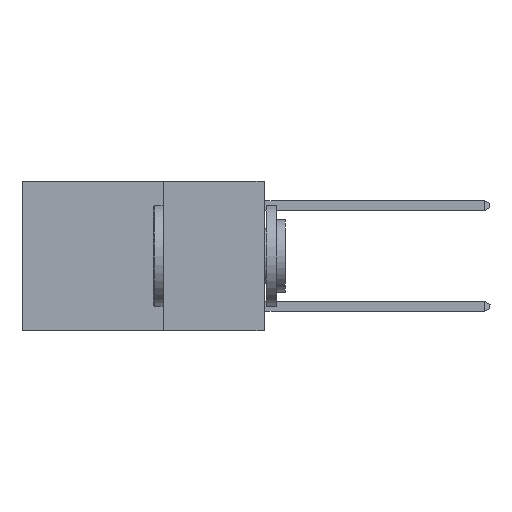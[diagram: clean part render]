
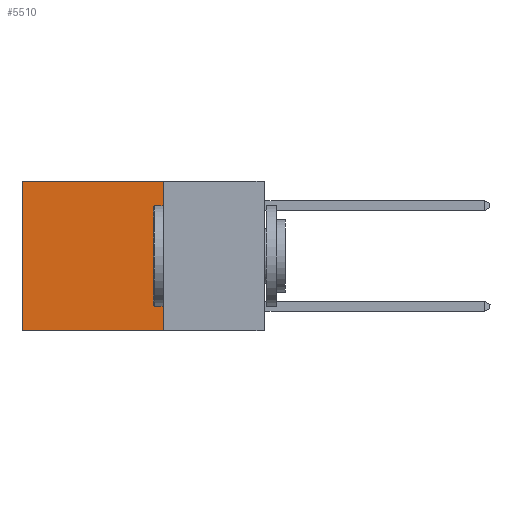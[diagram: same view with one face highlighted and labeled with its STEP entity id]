
A CAD part, left-side view. The second image highlights one B-rep face of the part: STEP entity #5510.
In plain terms, the highlighted planar face has unit normal (-1, 0, 0).
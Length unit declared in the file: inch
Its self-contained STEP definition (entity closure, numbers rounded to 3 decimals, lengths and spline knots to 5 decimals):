
#322 = PLANE ( 'NONE',  #14041 ) ;
#1677 = FACE_OUTER_BOUND ( 'NONE', #2921, .T. ) ;
#2061 = LINE ( 'NONE', #19884, #17164 ) ;
#2198 = CARTESIAN_POINT ( 'NONE',  ( 0.2625, 0.6, 0. ) ) ;
#2349 = DIRECTION ( 'NONE',  ( 1., 0., 0. ) ) ;
#2921 = EDGE_LOOP ( 'NONE', ( #15469, #20787, #21794, #24201 ) ) ;
#4219 = DIRECTION ( 'NONE',  ( 0., 0., -1. ) ) ;
#4571 = CARTESIAN_POINT ( 'NONE',  ( 0.2625, 0.25, -0.37 ) ) ;
#5058 = CARTESIAN_POINT ( 'NONE',  ( 0.2625, 0.25, 0. ) ) ;
#5510 = ADVANCED_FACE ( 'NONE', ( #1677 ), #322, .F. ) ;
#7798 = EDGE_CURVE ( 'NONE', #25427, #16414, #9970, .T. ) ;
#8755 = VECTOR ( 'NONE', #15962, 39.37008 ) ;
#9359 = EDGE_CURVE ( 'NONE', #24143, #25427, #21315, .T. ) ;
#9481 = DIRECTION ( 'NONE',  ( 0., 1., 0. ) ) ;
#9970 = LINE ( 'NONE', #2198, #8755 ) ;
#10730 = LINE ( 'NONE', #19510, #15329 ) ;
#14041 = AXIS2_PLACEMENT_3D ( 'NONE', #14146, #2349, #16122 ) ;
#14146 = CARTESIAN_POINT ( 'NONE',  ( 0.2625, 0.25, 0. ) ) ;
#14403 = CARTESIAN_POINT ( 'NONE',  ( 0.2625, 0.6, 0. ) ) ;
#15329 = VECTOR ( 'NONE', #21488, 39.37008 ) ;
#15469 = ORIENTED_EDGE ( 'NONE', *, *, #7798, .T. ) ;
#15962 = DIRECTION ( 'NONE',  ( 0., 0., -1. ) ) ;
#16122 = DIRECTION ( 'NONE',  ( 0., 0., -1. ) ) ;
#16414 = VERTEX_POINT ( 'NONE', #21299 ) ;
#17164 = VECTOR ( 'NONE', #4219, 39.37008 ) ;
#17916 = VECTOR ( 'NONE', #9481, 39.37008 ) ;
#19510 = CARTESIAN_POINT ( 'NONE',  ( 0.2625, 0.25, -0.37 ) ) ;
#19884 = CARTESIAN_POINT ( 'NONE',  ( 0.2625, 0.25, 0. ) ) ;
#20787 = ORIENTED_EDGE ( 'NONE', *, *, #24397, .F. ) ;
#21299 = CARTESIAN_POINT ( 'NONE',  ( 0.2625, 0.6, -0.37 ) ) ;
#21315 = LINE ( 'NONE', #23254, #17916 ) ;
#21488 = DIRECTION ( 'NONE',  ( 0., 1., 0. ) ) ;
#21794 = ORIENTED_EDGE ( 'NONE', *, *, #24725, .F. ) ;
#23254 = CARTESIAN_POINT ( 'NONE',  ( 0.2625, 0.25, 0. ) ) ;
#23430 = VERTEX_POINT ( 'NONE', #4571 ) ;
#24143 = VERTEX_POINT ( 'NONE', #5058 ) ;
#24201 = ORIENTED_EDGE ( 'NONE', *, *, #9359, .T. ) ;
#24397 = EDGE_CURVE ( 'NONE', #23430, #16414, #10730, .T. ) ;
#24725 = EDGE_CURVE ( 'NONE', #24143, #23430, #2061, .T. ) ;
#25427 = VERTEX_POINT ( 'NONE', #14403 ) ;
